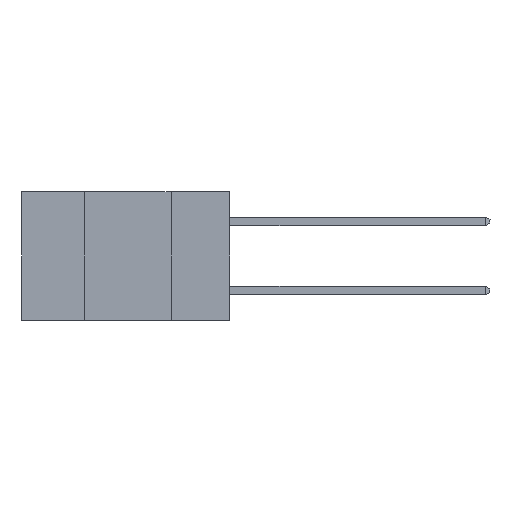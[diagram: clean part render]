
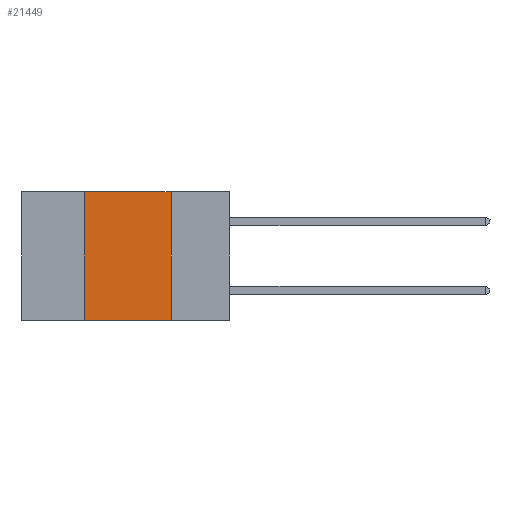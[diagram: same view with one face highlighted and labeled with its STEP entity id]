
A CAD part, left-side view. The second image highlights one B-rep face of the part: STEP entity #21449.
In plain terms, the highlighted planar face has unit normal (-1, 0, 0).
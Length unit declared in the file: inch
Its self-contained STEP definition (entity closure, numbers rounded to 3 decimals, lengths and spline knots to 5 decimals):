
#232 = LINE ( 'NONE', #15397, #11618 ) ;
#1305 = VERTEX_POINT ( 'NONE', #7355 ) ;
#1890 = EDGE_LOOP ( 'NONE', ( #26374, #9033, #2561, #9750 ) ) ;
#2561 = ORIENTED_EDGE ( 'NONE', *, *, #27286, .F. ) ;
#3262 = EDGE_CURVE ( 'NONE', #17204, #14391, #3754, .T. ) ;
#3754 = LINE ( 'NONE', #8159, #27030 ) ;
#4711 = CARTESIAN_POINT ( 'NONE',  ( 0., 0.42, 0. ) ) ;
#4964 = AXIS2_PLACEMENT_3D ( 'NONE', #20354, #6841, #22661 ) ;
#6556 = VECTOR ( 'NONE', #28609, 39.37008 ) ;
#6677 = VERTEX_POINT ( 'NONE', #19568 ) ;
#6841 = DIRECTION ( 'NONE',  ( 1., 0., 0. ) ) ;
#6944 = DIRECTION ( 'NONE',  ( 0., 0., 1. ) ) ;
#7355 = CARTESIAN_POINT ( 'NONE',  ( 0., 0.42, 0. ) ) ;
#8159 = CARTESIAN_POINT ( 'NONE',  ( 0., 0.17, 0. ) ) ;
#9033 = ORIENTED_EDGE ( 'NONE', *, *, #16977, .F. ) ;
#9693 = FACE_OUTER_BOUND ( 'NONE', #1890, .T. ) ;
#9750 = ORIENTED_EDGE ( 'NONE', *, *, #13837, .T. ) ;
#11125 = LINE ( 'NONE', #26394, #6556 ) ;
#11141 = DIRECTION ( 'NONE',  ( 0., 0., -1. ) ) ;
#11618 = VECTOR ( 'NONE', #28897, 39.37008 ) ;
#13542 = PLANE ( 'NONE',  #4964 ) ;
#13837 = EDGE_CURVE ( 'NONE', #6677, #14391, #232, .T. ) ;
#14391 = VERTEX_POINT ( 'NONE', #21626 ) ;
#15397 = CARTESIAN_POINT ( 'NONE',  ( 0., 0.6, -0.37 ) ) ;
#16125 = LINE ( 'NONE', #4711, #27392 ) ;
#16977 = EDGE_CURVE ( 'NONE', #1305, #17204, #11125, .T. ) ;
#17204 = VERTEX_POINT ( 'NONE', #18057 ) ;
#18057 = CARTESIAN_POINT ( 'NONE',  ( 0., 0.17, 0. ) ) ;
#19568 = CARTESIAN_POINT ( 'NONE',  ( 0., 0.42, -0.37 ) ) ;
#20354 = CARTESIAN_POINT ( 'NONE',  ( 0., 0.6, 0. ) ) ;
#21449 = ADVANCED_FACE ( 'NONE', ( #9693 ), #13542, .F. ) ;
#21626 = CARTESIAN_POINT ( 'NONE',  ( 0., 0.17, -0.37 ) ) ;
#22661 = DIRECTION ( 'NONE',  ( 0., 0., -1. ) ) ;
#26374 = ORIENTED_EDGE ( 'NONE', *, *, #3262, .F. ) ;
#26394 = CARTESIAN_POINT ( 'NONE',  ( 0., 0.6, 0. ) ) ;
#27030 = VECTOR ( 'NONE', #11141, 39.37008 ) ;
#27286 = EDGE_CURVE ( 'NONE', #6677, #1305, #16125, .T. ) ;
#27392 = VECTOR ( 'NONE', #6944, 39.37008 ) ;
#28609 = DIRECTION ( 'NONE',  ( 0., -1., 0. ) ) ;
#28897 = DIRECTION ( 'NONE',  ( 0., -1., 0. ) ) ;
